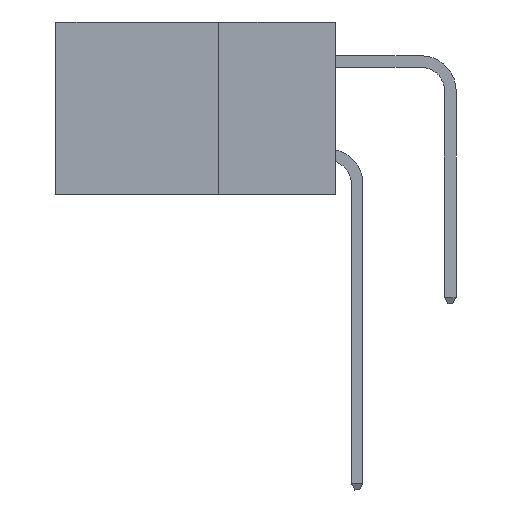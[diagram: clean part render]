
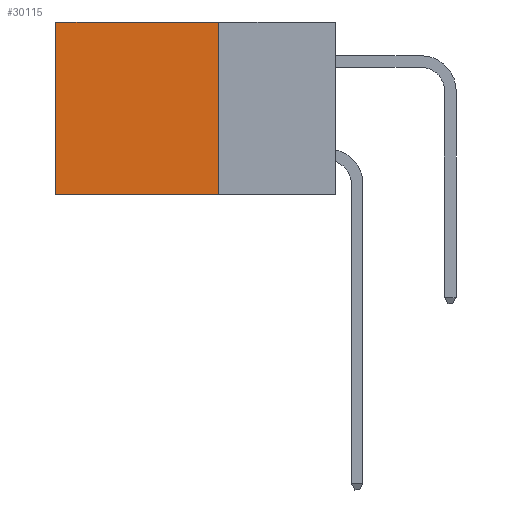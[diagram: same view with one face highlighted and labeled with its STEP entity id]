
A CAD part, left-side view. The second image highlights one B-rep face of the part: STEP entity #30115.
In plain terms, the highlighted planar face has unit normal (-1, 0, 0).
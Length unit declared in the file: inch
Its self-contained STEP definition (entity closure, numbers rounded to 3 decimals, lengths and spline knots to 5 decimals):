
#965 = VECTOR ( 'NONE', #27614, 39.37008 ) ;
#1053 = ORIENTED_EDGE ( 'NONE', *, *, #28000, .T. ) ;
#2706 = LINE ( 'NONE', #10154, #26744 ) ;
#3124 = EDGE_CURVE ( 'NONE', #8855, #19565, #24980, .T. ) ;
#4705 = CARTESIAN_POINT ( 'NONE',  ( 0.2875, 0.6, 0. ) ) ;
#5217 = DIRECTION ( 'NONE',  ( 1., 0., 0. ) ) ;
#6150 = DIRECTION ( 'NONE',  ( 0., 1., 0. ) ) ;
#6290 = CARTESIAN_POINT ( 'NONE',  ( 0.2875, 0.25, 0. ) ) ;
#7336 = VECTOR ( 'NONE', #6150, 39.37008 ) ;
#7671 = PLANE ( 'NONE',  #23194 ) ;
#8855 = VERTEX_POINT ( 'NONE', #4705 ) ;
#10154 = CARTESIAN_POINT ( 'NONE',  ( 0.2875, 0.25, 0. ) ) ;
#10425 = CARTESIAN_POINT ( 'NONE',  ( 0.2875, 0.25, -0.37 ) ) ;
#12036 = EDGE_CURVE ( 'NONE', #21633, #29721, #12560, .T. ) ;
#12560 = LINE ( 'NONE', #6290, #17989 ) ;
#12582 = CARTESIAN_POINT ( 'NONE',  ( 0.2875, 0.6, -0.37 ) ) ;
#13176 = CARTESIAN_POINT ( 'NONE',  ( 0.2875, 0.25, -0.37 ) ) ;
#13927 = DIRECTION ( 'NONE',  ( 0., 1., 0. ) ) ;
#16074 = CARTESIAN_POINT ( 'NONE',  ( 0.2875, 0.6, 0. ) ) ;
#16689 = CARTESIAN_POINT ( 'NONE',  ( 0.2875, 0.25, 0. ) ) ;
#17659 = DIRECTION ( 'NONE',  ( 0., 0., -1. ) ) ;
#17868 = FACE_OUTER_BOUND ( 'NONE', #20500, .T. ) ;
#17989 = VECTOR ( 'NONE', #17659, 39.37008 ) ;
#19565 = VERTEX_POINT ( 'NONE', #12582 ) ;
#20384 = ORIENTED_EDGE ( 'NONE', *, *, #27326, .F. ) ;
#20500 = EDGE_LOOP ( 'NONE', ( #27170, #20384, #22420, #1053 ) ) ;
#21491 = LINE ( 'NONE', #10425, #7336 ) ;
#21633 = VERTEX_POINT ( 'NONE', #16689 ) ;
#22420 = ORIENTED_EDGE ( 'NONE', *, *, #12036, .F. ) ;
#23194 = AXIS2_PLACEMENT_3D ( 'NONE', #28604, #5217, #26360 ) ;
#24980 = LINE ( 'NONE', #16074, #965 ) ;
#26360 = DIRECTION ( 'NONE',  ( 0., 0., -1. ) ) ;
#26744 = VECTOR ( 'NONE', #13927, 39.37008 ) ;
#27170 = ORIENTED_EDGE ( 'NONE', *, *, #3124, .T. ) ;
#27326 = EDGE_CURVE ( 'NONE', #29721, #19565, #21491, .T. ) ;
#27614 = DIRECTION ( 'NONE',  ( 0., 0., -1. ) ) ;
#28000 = EDGE_CURVE ( 'NONE', #21633, #8855, #2706, .T. ) ;
#28604 = CARTESIAN_POINT ( 'NONE',  ( 0.2875, 0.25, 0. ) ) ;
#29721 = VERTEX_POINT ( 'NONE', #13176 ) ;
#30115 = ADVANCED_FACE ( 'NONE', ( #17868 ), #7671, .F. ) ;
